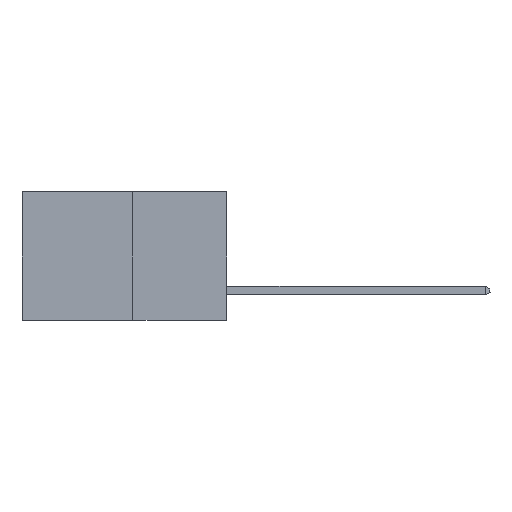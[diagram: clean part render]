
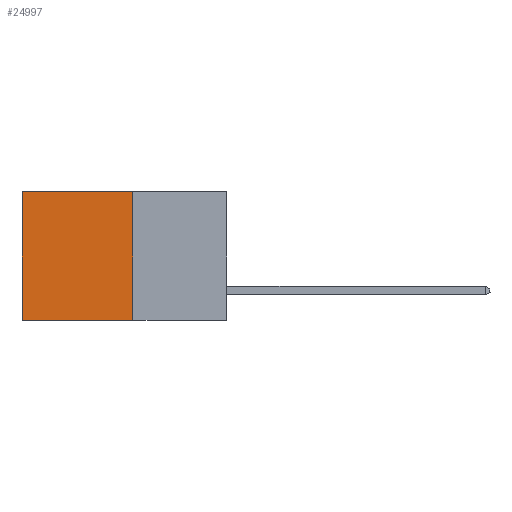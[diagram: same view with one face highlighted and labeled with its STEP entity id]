
A CAD part, left-side view. The second image highlights one B-rep face of the part: STEP entity #24997.
In plain terms, the highlighted planar face has unit normal (-1, 0, 0).
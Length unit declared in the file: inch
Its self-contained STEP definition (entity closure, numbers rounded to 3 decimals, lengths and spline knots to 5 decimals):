
#200 = CARTESIAN_POINT ( 'NONE',  ( 0.277, 0.27, 0. ) ) ;
#595 = DIRECTION ( 'NONE',  ( 0., 0., -1. ) ) ;
#652 = LINE ( 'NONE', #5500, #6365 ) ;
#1027 = VERTEX_POINT ( 'NONE', #17930 ) ;
#1252 = CARTESIAN_POINT ( 'NONE',  ( 0.277, 0.27, -0.37 ) ) ;
#1882 = DIRECTION ( 'NONE',  ( 0., 1., 0. ) ) ;
#4814 = VERTEX_POINT ( 'NONE', #200 ) ;
#5500 = CARTESIAN_POINT ( 'NONE',  ( 0.277, 0.27, -0.37 ) ) ;
#5853 = DIRECTION ( 'NONE',  ( 0., 0., -1. ) ) ;
#5872 = EDGE_CURVE ( 'NONE', #6391, #1027, #27291, .T. ) ;
#5984 = FACE_OUTER_BOUND ( 'NONE', #18282, .T. ) ;
#6365 = VECTOR ( 'NONE', #5853, 39.37008 ) ;
#6391 = VERTEX_POINT ( 'NONE', #21449 ) ;
#7595 = EDGE_CURVE ( 'NONE', #4814, #15457, #652, .T. ) ;
#8510 = ORIENTED_EDGE ( 'NONE', *, *, #7595, .F. ) ;
#9686 = LINE ( 'NONE', #14070, #15409 ) ;
#11312 = ORIENTED_EDGE ( 'NONE', *, *, #14964, .T. ) ;
#14070 = CARTESIAN_POINT ( 'NONE',  ( 0.277, 0.27, -0.37 ) ) ;
#14964 = EDGE_CURVE ( 'NONE', #4814, #6391, #28182, .T. ) ;
#15206 = DIRECTION ( 'NONE',  ( 1., 0., 0. ) ) ;
#15409 = VECTOR ( 'NONE', #1882, 39.37008 ) ;
#15457 = VERTEX_POINT ( 'NONE', #1252 ) ;
#16138 = VECTOR ( 'NONE', #28459, 39.37008 ) ;
#17468 = CARTESIAN_POINT ( 'NONE',  ( 0.277, 0.27, -0.37 ) ) ;
#17930 = CARTESIAN_POINT ( 'NONE',  ( 0.277, 0.59, -0.37 ) ) ;
#18282 = EDGE_LOOP ( 'NONE', ( #27322, #27549, #8510, #11312 ) ) ;
#20881 = EDGE_CURVE ( 'NONE', #15457, #1027, #9686, .T. ) ;
#21449 = CARTESIAN_POINT ( 'NONE',  ( 0.277, 0.59, 0. ) ) ;
#24997 = ADVANCED_FACE ( 'NONE', ( #5984 ), #29547, .F. ) ;
#26557 = VECTOR ( 'NONE', #28581, 39.37008 ) ;
#27291 = LINE ( 'NONE', #28496, #26557 ) ;
#27322 = ORIENTED_EDGE ( 'NONE', *, *, #5872, .T. ) ;
#27549 = ORIENTED_EDGE ( 'NONE', *, *, #20881, .F. ) ;
#27805 = AXIS2_PLACEMENT_3D ( 'NONE', #17468, #15206, #595 ) ;
#28182 = LINE ( 'NONE', #30839, #16138 ) ;
#28459 = DIRECTION ( 'NONE',  ( 0., 1., 0. ) ) ;
#28496 = CARTESIAN_POINT ( 'NONE',  ( 0.277, 0.59, -0.37 ) ) ;
#28581 = DIRECTION ( 'NONE',  ( 0., 0., -1. ) ) ;
#29547 = PLANE ( 'NONE',  #27805 ) ;
#30839 = CARTESIAN_POINT ( 'NONE',  ( 0.277, 0.27, 0. ) ) ;
